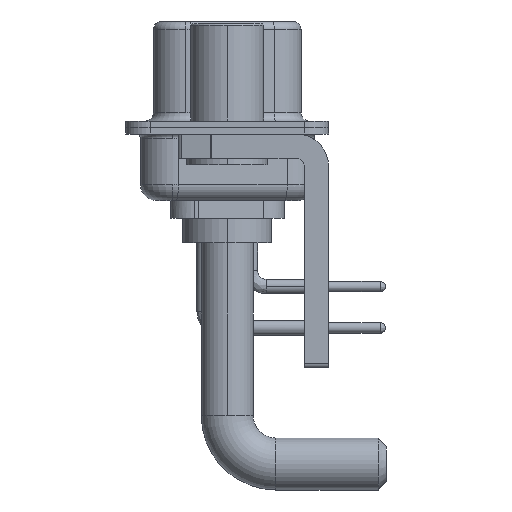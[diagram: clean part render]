
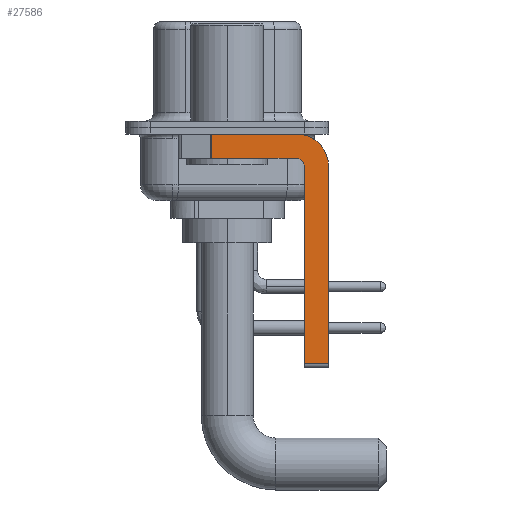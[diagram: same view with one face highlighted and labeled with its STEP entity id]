
A CAD part, left-side view. The second image highlights one B-rep face of the part: STEP entity #27586.
In plain terms, the highlighted planar face has unit normal (-1, 0, 0).
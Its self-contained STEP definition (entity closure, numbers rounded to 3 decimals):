
#508 = VECTOR ( 'NONE', #4865, 1000. ) ;
#511 = CARTESIAN_POINT ( 'NONE',  ( -2.9, -6.25, -14.55 ) ) ;
#608 = VERTEX_POINT ( 'NONE', #24169 ) ;
#700 = CIRCLE ( 'NONE', #29076, 0.5 ) ;
#767 = CARTESIAN_POINT ( 'NONE',  ( -2.9, 3., -0.4 ) ) ;
#1204 = DIRECTION ( 'NONE',  ( 0., 0., -1. ) ) ;
#2307 = EDGE_CURVE ( 'NONE', #608, #12816, #6984, .T. ) ;
#2462 = CARTESIAN_POINT ( 'NONE',  ( -2.9, 0.978, -0.4 ) ) ;
#2916 = ORIENTED_EDGE ( 'NONE', *, *, #6922, .F. ) ;
#3227 = EDGE_CURVE ( 'NONE', #17098, #608, #14510, .T. ) ;
#4865 = DIRECTION ( 'NONE',  ( 0., 1., 0. ) ) ;
#5461 = EDGE_CURVE ( 'NONE', #28131, #17763, #700, .T. ) ;
#5647 = DIRECTION ( 'NONE',  ( 0., -1., 0. ) ) ;
#6064 = DIRECTION ( 'NONE',  ( 0., -1., 0. ) ) ;
#6801 = CARTESIAN_POINT ( 'NONE',  ( -2.9, -4.25, -2.4 ) ) ;
#6922 = EDGE_CURVE ( 'NONE', #18504, #28131, #6973, .T. ) ;
#6973 = LINE ( 'NONE', #25032, #21084 ) ;
#6984 = CIRCLE ( 'NONE', #8843, 2. ) ;
#7693 = ORIENTED_EDGE ( 'NONE', *, *, #5461, .F. ) ;
#8400 = CARTESIAN_POINT ( 'NONE',  ( -2.9, -4.25, -2.4 ) ) ;
#8571 = CARTESIAN_POINT ( 'NONE',  ( -2.9, -4.25, -14.55 ) ) ;
#8843 = AXIS2_PLACEMENT_3D ( 'NONE', #14159, #18450, #13532 ) ;
#9343 = AXIS2_PLACEMENT_3D ( 'NONE', #8400, #17410, #12522 ) ;
#9363 = CARTESIAN_POINT ( 'NONE',  ( -2.9, -4.25, -1.9 ) ) ;
#9785 = CARTESIAN_POINT ( 'NONE',  ( -2.9, -6.25, -2.4 ) ) ;
#10271 = ORIENTED_EDGE ( 'NONE', *, *, #22635, .T. ) ;
#10369 = LINE ( 'NONE', #9785, #20742 ) ;
#10975 = EDGE_CURVE ( 'NONE', #17098, #13549, #16323, .T. ) ;
#11266 = VECTOR ( 'NONE', #1204, 1000. ) ;
#12522 = DIRECTION ( 'NONE',  ( 0., 0., -1. ) ) ;
#12813 = PLANE ( 'NONE',  #9343 ) ;
#12816 = VERTEX_POINT ( 'NONE', #14014 ) ;
#13062 = CARTESIAN_POINT ( 'NONE',  ( -2.9, -4.75, -2.4 ) ) ;
#13284 = ORIENTED_EDGE ( 'NONE', *, *, #15121, .F. ) ;
#13395 = CARTESIAN_POINT ( 'NONE',  ( -2.9, -4.25, -1.9 ) ) ;
#13532 = DIRECTION ( 'NONE',  ( 0., 0., -1. ) ) ;
#13549 = VERTEX_POINT ( 'NONE', #27689 ) ;
#14014 = CARTESIAN_POINT ( 'NONE',  ( -2.9, -6.25, -2.4 ) ) ;
#14159 = CARTESIAN_POINT ( 'NONE',  ( -2.9, -4.25, -2.4 ) ) ;
#14210 = CARTESIAN_POINT ( 'NONE',  ( -2.9, -4.75, -14.55 ) ) ;
#14510 = LINE ( 'NONE', #767, #23612 ) ;
#15121 = EDGE_CURVE ( 'NONE', #17763, #13549, #27081, .T. ) ;
#15794 = DIRECTION ( 'NONE',  ( -1., 0., 0. ) ) ;
#15796 = EDGE_LOOP ( 'NONE', ( #28609, #22329, #13284, #7693, #2916, #10271, #19916, #21348 ) ) ;
#16243 = DIRECTION ( 'NONE',  ( 0., 0., 1. ) ) ;
#16323 = LINE ( 'NONE', #25241, #11266 ) ;
#17098 = VERTEX_POINT ( 'NONE', #2462 ) ;
#17410 = DIRECTION ( 'NONE',  ( 1., 0., 0. ) ) ;
#17763 = VERTEX_POINT ( 'NONE', #9363 ) ;
#18450 = DIRECTION ( 'NONE',  ( 1., 0., 0. ) ) ;
#18504 = VERTEX_POINT ( 'NONE', #14210 ) ;
#19628 = FACE_OUTER_BOUND ( 'NONE', #15796, .T. ) ;
#19916 = ORIENTED_EDGE ( 'NONE', *, *, #28807, .F. ) ;
#20742 = VECTOR ( 'NONE', #25659, 1000. ) ;
#21084 = VECTOR ( 'NONE', #23108, 1000. ) ;
#21348 = ORIENTED_EDGE ( 'NONE', *, *, #2307, .F. ) ;
#22329 = ORIENTED_EDGE ( 'NONE', *, *, #10975, .T. ) ;
#22635 = EDGE_CURVE ( 'NONE', #18504, #25332, #28887, .T. ) ;
#23108 = DIRECTION ( 'NONE',  ( 0., 0., 1. ) ) ;
#23612 = VECTOR ( 'NONE', #5647, 1000. ) ;
#24169 = CARTESIAN_POINT ( 'NONE',  ( -2.9, -4.25, -0.4 ) ) ;
#25032 = CARTESIAN_POINT ( 'NONE',  ( -2.9, -4.75, -14.8 ) ) ;
#25241 = CARTESIAN_POINT ( 'NONE',  ( -2.9, 0.978, -1.9 ) ) ;
#25332 = VERTEX_POINT ( 'NONE', #511 ) ;
#25659 = DIRECTION ( 'NONE',  ( 0., 0., -1. ) ) ;
#26357 = VECTOR ( 'NONE', #6064, 1000. ) ;
#27081 = LINE ( 'NONE', #13395, #508 ) ;
#27586 = ADVANCED_FACE ( 'NONE', ( #19628 ), #12813, .F. ) ;
#27689 = CARTESIAN_POINT ( 'NONE',  ( -2.9, 0.978, -1.9 ) ) ;
#28131 = VERTEX_POINT ( 'NONE', #13062 ) ;
#28609 = ORIENTED_EDGE ( 'NONE', *, *, #3227, .F. ) ;
#28807 = EDGE_CURVE ( 'NONE', #12816, #25332, #10369, .T. ) ;
#28887 = LINE ( 'NONE', #8571, #26357 ) ;
#29076 = AXIS2_PLACEMENT_3D ( 'NONE', #6801, #15794, #16243 ) ;
